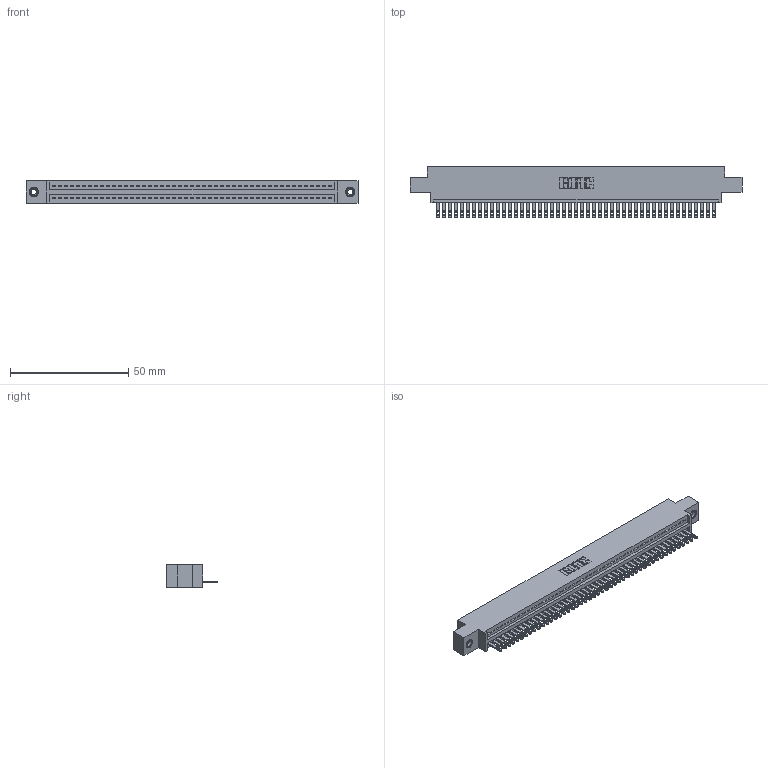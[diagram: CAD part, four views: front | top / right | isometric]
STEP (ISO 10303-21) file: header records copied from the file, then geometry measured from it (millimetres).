
FILE_DESCRIPTION (( 'STEP AP203' ), '1' );
FILE_NAME ('895-047-500-608.STEP', '2020-09-27T06:07:27', ( '' ), ( '' ), 'SwSTEP 2.0', 'SolidWorks 2020', '' );
FILE_SCHEMA (( 'CONFIG_CONTROL_DESIGN' ));
Length unit declared in the file: inch
Products named in the file (4): 895-047-500-608; 345-250-001_345-250-003-102; 345-292-001_345-293-100; 845 Part_0.170 Offset - 0.156 Dia-TI
Assembly tree (50 placements, depth 2):
  895-047-500-608
    845 Part_0.170 Offset - 0.156 Dia-TI
    345-292-001_345-293-100  x47
    345-250-001_345-250-003-102  x2
Bounding box: 140.59 x 21.51 x 9.4 mm (x, y, z)
Volume: 13303.4 mm3; surface area: 17998.3 mm2
Topology: 50 solids, 50 shells, 2728 faces, 8385 edges, 5582 vertices
Faces by surface type: plane 1714, cylinder 998, cone 12, torus 4
Entity records: 35948 total; most frequent: CARTESIAN_POINT 6208, ORIENTED_EDGE 6182, DIRECTION 5443, EDGE_CURVE 3091, LINE 2747, VECTOR 2747, VERTEX_POINT 2056, AXIS2_PLACEMENT_3D 1348
